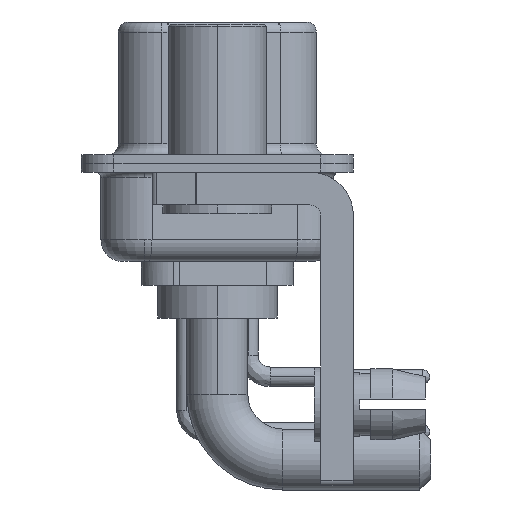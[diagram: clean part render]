
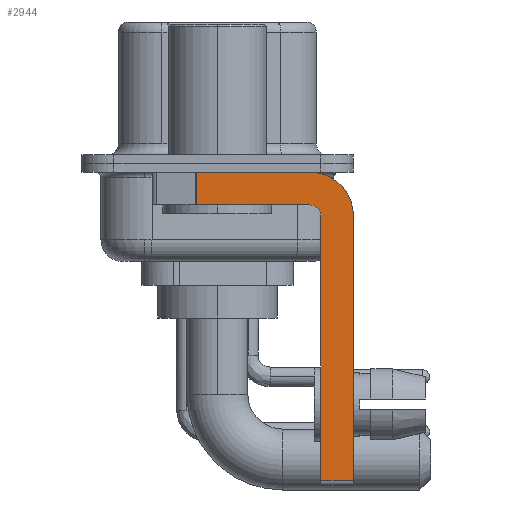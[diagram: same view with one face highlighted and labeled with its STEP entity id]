
A CAD part, left-side view. The second image highlights one B-rep face of the part: STEP entity #2944.
In plain terms, the highlighted planar face has unit normal (-1, 0, 0).
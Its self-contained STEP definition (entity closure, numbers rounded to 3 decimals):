
#42 = CARTESIAN_POINT ( 'NONE',  ( -2.9, -4.75, -14.55 ) ) ;
#182 = CARTESIAN_POINT ( 'NONE',  ( -2.9, -4.75, -2.4 ) ) ;
#278 = VECTOR ( 'NONE', #835, 1000. ) ;
#499 = LINE ( 'NONE', #12778, #31260 ) ;
#835 = DIRECTION ( 'NONE',  ( 0., -1., 0. ) ) ;
#1223 = AXIS2_PLACEMENT_3D ( 'NONE', #13925, #20916, #3722 ) ;
#1240 = ORIENTED_EDGE ( 'NONE', *, *, #11551, .F. ) ;
#1597 = ORIENTED_EDGE ( 'NONE', *, *, #3330, .F. ) ;
#2473 = AXIS2_PLACEMENT_3D ( 'NONE', #24467, #18968, #2660 ) ;
#2660 = DIRECTION ( 'NONE',  ( 0., 0., -1. ) ) ;
#2944 = ADVANCED_FACE ( 'NONE', ( #22539 ), #27930, .F. ) ;
#3015 = VECTOR ( 'NONE', #8274, 1000. ) ;
#3330 = EDGE_CURVE ( 'NONE', #11594, #9681, #20561, .T. ) ;
#3461 = ORIENTED_EDGE ( 'NONE', *, *, #12917, .T. ) ;
#3722 = DIRECTION ( 'NONE',  ( 0., 0., -1. ) ) ;
#4024 = EDGE_CURVE ( 'NONE', #11655, #17271, #29922, .T. ) ;
#4560 = CARTESIAN_POINT ( 'NONE',  ( -2.9, -6.25, -2.4 ) ) ;
#5191 = EDGE_CURVE ( 'NONE', #26314, #11594, #30598, .T. ) ;
#5450 = LINE ( 'NONE', #7996, #278 ) ;
#6807 = VERTEX_POINT ( 'NONE', #27959 ) ;
#7996 = CARTESIAN_POINT ( 'NONE',  ( -2.9, 3., -0.4 ) ) ;
#8274 = DIRECTION ( 'NONE',  ( 0., 0., -1. ) ) ;
#8442 = CARTESIAN_POINT ( 'NONE',  ( -2.9, 0.978, -1.9 ) ) ;
#8780 = LINE ( 'NONE', #30582, #14014 ) ;
#8878 = ORIENTED_EDGE ( 'NONE', *, *, #25118, .F. ) ;
#9496 = DIRECTION ( 'NONE',  ( 0., 0., -1. ) ) ;
#9681 = VERTEX_POINT ( 'NONE', #14880 ) ;
#10403 = VERTEX_POINT ( 'NONE', #30739 ) ;
#11551 = EDGE_CURVE ( 'NONE', #9681, #16171, #499, .T. ) ;
#11594 = VERTEX_POINT ( 'NONE', #182 ) ;
#11655 = VERTEX_POINT ( 'NONE', #15317 ) ;
#12778 = CARTESIAN_POINT ( 'NONE',  ( -2.9, -4.25, -1.9 ) ) ;
#12917 = EDGE_CURVE ( 'NONE', #26314, #10403, #8780, .T. ) ;
#13925 = CARTESIAN_POINT ( 'NONE',  ( -2.9, -4.25, -2.4 ) ) ;
#14014 = VECTOR ( 'NONE', #20726, 1000. ) ;
#14880 = CARTESIAN_POINT ( 'NONE',  ( -2.9, -4.25, -1.9 ) ) ;
#15108 = ORIENTED_EDGE ( 'NONE', *, *, #18966, .F. ) ;
#15317 = CARTESIAN_POINT ( 'NONE',  ( -2.9, -4.25, -0.4 ) ) ;
#15484 = DIRECTION ( 'NONE',  ( -1., 0., 0. ) ) ;
#16171 = VERTEX_POINT ( 'NONE', #20696 ) ;
#16247 = EDGE_CURVE ( 'NONE', #6807, #16171, #22763, .T. ) ;
#16983 = LINE ( 'NONE', #4560, #26040 ) ;
#17271 = VERTEX_POINT ( 'NONE', #28912 ) ;
#17549 = CARTESIAN_POINT ( 'NONE',  ( -2.9, -4.25, -2.4 ) ) ;
#18966 = EDGE_CURVE ( 'NONE', #17271, #10403, #16983, .T. ) ;
#18968 = DIRECTION ( 'NONE',  ( 1., 0., 0. ) ) ;
#19347 = VECTOR ( 'NONE', #28060, 1000. ) ;
#20561 = CIRCLE ( 'NONE', #22589, 0.5 ) ;
#20696 = CARTESIAN_POINT ( 'NONE',  ( -2.9, 0.978, -1.9 ) ) ;
#20726 = DIRECTION ( 'NONE',  ( 0., -1., 0. ) ) ;
#20916 = DIRECTION ( 'NONE',  ( 1., 0., 0. ) ) ;
#22153 = DIRECTION ( 'NONE',  ( 0., 0., 1. ) ) ;
#22539 = FACE_OUTER_BOUND ( 'NONE', #28286, .T. ) ;
#22589 = AXIS2_PLACEMENT_3D ( 'NONE', #17549, #15484, #22153 ) ;
#22763 = LINE ( 'NONE', #8442, #3015 ) ;
#24467 = CARTESIAN_POINT ( 'NONE',  ( -2.9, -4.25, -2.4 ) ) ;
#25009 = DIRECTION ( 'NONE',  ( 0., 1., 0. ) ) ;
#25118 = EDGE_CURVE ( 'NONE', #6807, #11655, #5450, .T. ) ;
#25611 = ORIENTED_EDGE ( 'NONE', *, *, #4024, .F. ) ;
#26040 = VECTOR ( 'NONE', #9496, 1000. ) ;
#26314 = VERTEX_POINT ( 'NONE', #42 ) ;
#26839 = ORIENTED_EDGE ( 'NONE', *, *, #16247, .T. ) ;
#27930 = PLANE ( 'NONE',  #1223 ) ;
#27959 = CARTESIAN_POINT ( 'NONE',  ( -2.9, 0.978, -0.4 ) ) ;
#28060 = DIRECTION ( 'NONE',  ( 0., 0., 1. ) ) ;
#28286 = EDGE_LOOP ( 'NONE', ( #8878, #26839, #1240, #1597, #29746, #3461, #15108, #25611 ) ) ;
#28912 = CARTESIAN_POINT ( 'NONE',  ( -2.9, -6.25, -2.4 ) ) ;
#29746 = ORIENTED_EDGE ( 'NONE', *, *, #5191, .F. ) ;
#29922 = CIRCLE ( 'NONE', #2473, 2. ) ;
#30582 = CARTESIAN_POINT ( 'NONE',  ( -2.9, -4.25, -14.55 ) ) ;
#30598 = LINE ( 'NONE', #30910, #19347 ) ;
#30739 = CARTESIAN_POINT ( 'NONE',  ( -2.9, -6.25, -14.55 ) ) ;
#30910 = CARTESIAN_POINT ( 'NONE',  ( -2.9, -4.75, -14.8 ) ) ;
#31260 = VECTOR ( 'NONE', #25009, 1000. ) ;
